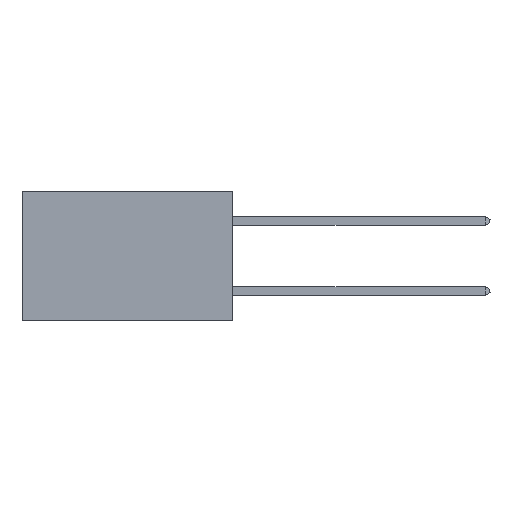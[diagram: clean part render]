
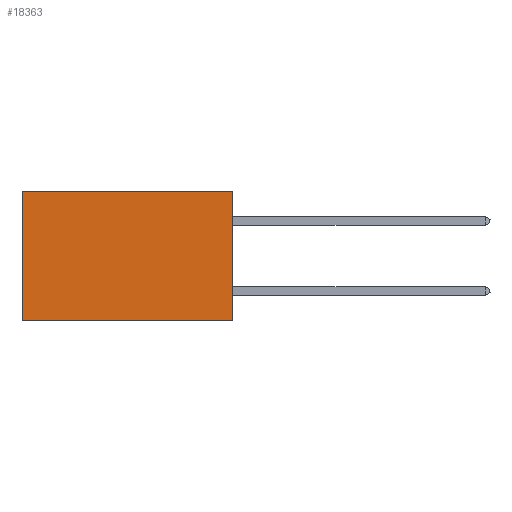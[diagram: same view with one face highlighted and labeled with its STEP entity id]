
A CAD part, left-side view. The second image highlights one B-rep face of the part: STEP entity #18363.
In plain terms, the highlighted planar face has unit normal (-1, 0, 0).
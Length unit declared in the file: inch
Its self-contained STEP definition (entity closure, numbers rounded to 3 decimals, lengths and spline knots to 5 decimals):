
#964 = CARTESIAN_POINT ( 'NONE',  ( 0.2875, 0., 0. ) ) ;
#1280 = VECTOR ( 'NONE', #31636, 39.37008 ) ;
#1494 = DIRECTION ( 'NONE',  ( 1., 0., 0. ) ) ;
#2385 = EDGE_CURVE ( 'NONE', #8543, #17870, #4348, .T. ) ;
#2553 = LINE ( 'NONE', #25820, #9306 ) ;
#3023 = DIRECTION ( 'NONE',  ( 0., 0., -1. ) ) ;
#3794 = VERTEX_POINT ( 'NONE', #17314 ) ;
#4341 = EDGE_LOOP ( 'NONE', ( #36475, #13978, #22884, #20692 ) ) ;
#4348 = LINE ( 'NONE', #26467, #15999 ) ;
#5189 = DIRECTION ( 'NONE',  ( 0., 1., 0. ) ) ;
#5688 = EDGE_CURVE ( 'NONE', #3794, #8543, #12161, .T. ) ;
#8543 = VERTEX_POINT ( 'NONE', #26748 ) ;
#8757 = CARTESIAN_POINT ( 'NONE',  ( 0.2875, 0., -0.37 ) ) ;
#9306 = VECTOR ( 'NONE', #3023, 39.37008 ) ;
#10524 = PLANE ( 'NONE',  #23401 ) ;
#12161 = LINE ( 'NONE', #964, #21508 ) ;
#13323 = FACE_OUTER_BOUND ( 'NONE', #4341, .T. ) ;
#13663 = VERTEX_POINT ( 'NONE', #21934 ) ;
#13978 = ORIENTED_EDGE ( 'NONE', *, *, #22626, .F. ) ;
#15999 = VECTOR ( 'NONE', #31832, 39.37008 ) ;
#16210 = EDGE_CURVE ( 'NONE', #3794, #13663, #2553, .T. ) ;
#17305 = CARTESIAN_POINT ( 'NONE',  ( 0.2875, 0.6, -0.37 ) ) ;
#17314 = CARTESIAN_POINT ( 'NONE',  ( 0.2875, 0., 0. ) ) ;
#17870 = VERTEX_POINT ( 'NONE', #17305 ) ;
#18363 = ADVANCED_FACE ( 'NONE', ( #13323 ), #10524, .F. ) ;
#18792 = CARTESIAN_POINT ( 'NONE',  ( 0.2875, 0., 0. ) ) ;
#20692 = ORIENTED_EDGE ( 'NONE', *, *, #5688, .T. ) ;
#21435 = LINE ( 'NONE', #8757, #1280 ) ;
#21508 = VECTOR ( 'NONE', #5189, 39.37008 ) ;
#21934 = CARTESIAN_POINT ( 'NONE',  ( 0.2875, 0., -0.37 ) ) ;
#22626 = EDGE_CURVE ( 'NONE', #13663, #17870, #21435, .T. ) ;
#22884 = ORIENTED_EDGE ( 'NONE', *, *, #16210, .F. ) ;
#23401 = AXIS2_PLACEMENT_3D ( 'NONE', #18792, #1494, #30153 ) ;
#25820 = CARTESIAN_POINT ( 'NONE',  ( 0.2875, 0., 0. ) ) ;
#26467 = CARTESIAN_POINT ( 'NONE',  ( 0.2875, 0.6, 0. ) ) ;
#26748 = CARTESIAN_POINT ( 'NONE',  ( 0.2875, 0.6, 0. ) ) ;
#30153 = DIRECTION ( 'NONE',  ( 0., 0., -1. ) ) ;
#31636 = DIRECTION ( 'NONE',  ( 0., 1., 0. ) ) ;
#31832 = DIRECTION ( 'NONE',  ( 0., 0., -1. ) ) ;
#36475 = ORIENTED_EDGE ( 'NONE', *, *, #2385, .T. ) ;
